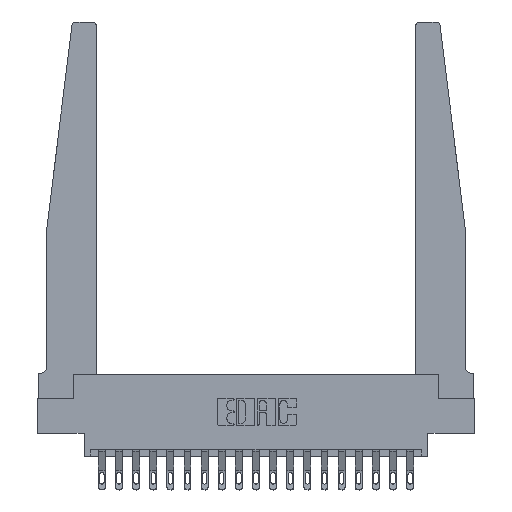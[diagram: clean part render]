
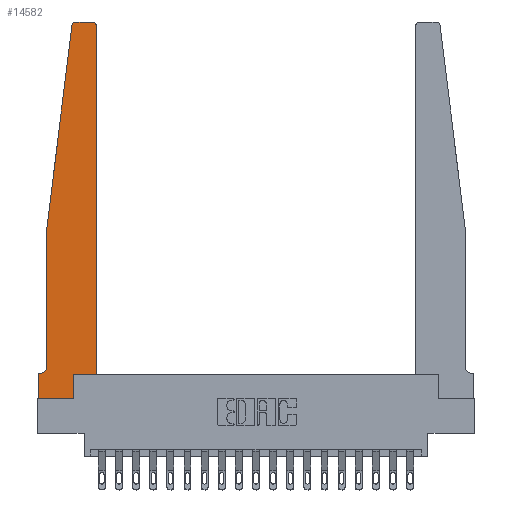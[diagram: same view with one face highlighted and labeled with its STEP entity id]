
A CAD part, top view. The second image highlights one B-rep face of the part: STEP entity #14582.
In plain terms, the highlighted planar face has unit normal (0, 0, 1).
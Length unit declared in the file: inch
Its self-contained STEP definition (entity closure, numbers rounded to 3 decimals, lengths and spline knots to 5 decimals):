
#494 = CARTESIAN_POINT ( 'NONE',  ( 0.425, 0.18, 0.37 ) ) ;
#512 = CARTESIAN_POINT ( 'NONE',  ( 0., 0., 0.37 ) ) ;
#1252 = CARTESIAN_POINT ( 'NONE',  ( 0.425, 0.18, 0.37 ) ) ;
#1759 = DIRECTION ( 'NONE',  ( 0., 1., 0. ) ) ;
#1803 = DIRECTION ( 'NONE',  ( 1., 0., 0. ) ) ;
#1852 = CARTESIAN_POINT ( 'NONE',  ( 0.2605, 0.18, 0.37 ) ) ;
#1976 = VERTEX_POINT ( 'NONE', #13450 ) ;
#2086 = DIRECTION ( 'NONE',  ( 0., 0., 1. ) ) ;
#2356 = VECTOR ( 'NONE', #1803, 39.37008 ) ;
#2367 = VECTOR ( 'NONE', #16394, 39.37008 ) ;
#2510 = DIRECTION ( 'NONE',  ( -1., 0., 0. ) ) ;
#2608 = CARTESIAN_POINT ( 'NONE',  ( 0.015, 0.2375, 0.37 ) ) ;
#2613 = VERTEX_POINT ( 'NONE', #1852 ) ;
#2911 = VERTEX_POINT ( 'NONE', #11051 ) ;
#3124 = ORIENTED_EDGE ( 'NONE', *, *, #18008, .T. ) ;
#3172 = CIRCLE ( 'NONE', #20982, 0.03 ) ;
#3353 = CARTESIAN_POINT ( 'NONE',  ( 0.065, 0.1875, 0.37 ) ) ;
#3414 = VERTEX_POINT ( 'NONE', #3780 ) ;
#3439 = ORIENTED_EDGE ( 'NONE', *, *, #6816, .T. ) ;
#3484 = EDGE_CURVE ( 'NONE', #9078, #5888, #3172, .T. ) ;
#3780 = CARTESIAN_POINT ( 'NONE',  ( 0.425, 0.18, 0.37 ) ) ;
#3910 = AXIS2_PLACEMENT_3D ( 'NONE', #19140, #8036, #21086 ) ;
#3924 = VECTOR ( 'NONE', #4923, 39.37008 ) ;
#3942 = CIRCLE ( 'NONE', #11148, 0.05 ) ;
#4830 = FACE_OUTER_BOUND ( 'NONE', #9101, .T. ) ;
#4867 = LINE ( 'NONE', #3353, #16237 ) ;
#4923 = DIRECTION ( 'NONE',  ( 0., -1., 0. ) ) ;
#5519 = VECTOR ( 'NONE', #19209, 39.37008 ) ;
#5888 = VERTEX_POINT ( 'NONE', #18949 ) ;
#6439 = ORIENTED_EDGE ( 'NONE', *, *, #17632, .T. ) ;
#6446 = PLANE ( 'NONE',  #6995 ) ;
#6758 = LINE ( 'NONE', #8273, #3924 ) ;
#6816 = EDGE_CURVE ( 'NONE', #17831, #2911, #14531, .T. ) ;
#6824 = VECTOR ( 'NONE', #8120, 39.37008 ) ;
#6889 = EDGE_CURVE ( 'NONE', #13131, #13969, #13159, .T. ) ;
#6995 = AXIS2_PLACEMENT_3D ( 'NONE', #12984, #9667, #11596 ) ;
#7030 = ORIENTED_EDGE ( 'NONE', *, *, #18365, .T. ) ;
#7770 = LINE ( 'NONE', #14387, #5519 ) ;
#7805 = DIRECTION ( 'NONE',  ( 0., 1., 0. ) ) ;
#8036 = DIRECTION ( 'NONE',  ( 0., 0., 1. ) ) ;
#8120 = DIRECTION ( 'NONE',  ( 0., -1., 0. ) ) ;
#8273 = CARTESIAN_POINT ( 'NONE',  ( 0.065, 1.25, 0.37 ) ) ;
#8353 = EDGE_CURVE ( 'NONE', #17542, #13131, #9708, .T. ) ;
#9044 = CARTESIAN_POINT ( 'NONE',  ( 0.425, 2.72, 0.37 ) ) ;
#9078 = VERTEX_POINT ( 'NONE', #9044 ) ;
#9101 = EDGE_LOOP ( 'NONE', ( #16746, #3439, #15639, #6439, #3124, #14637, #19939, #14296, #7030, #11857, #20374, #21070 ) ) ;
#9299 = EDGE_CURVE ( 'NONE', #2911, #1976, #10105, .T. ) ;
#9595 = DIRECTION ( 'NONE',  ( -1., 0., 0. ) ) ;
#9667 = DIRECTION ( 'NONE',  ( 0., 0., 1. ) ) ;
#9708 = LINE ( 'NONE', #17937, #6824 ) ;
#10077 = VERTEX_POINT ( 'NONE', #16934 ) ;
#10105 = LINE ( 'NONE', #12977, #2367 ) ;
#10882 = CARTESIAN_POINT ( 'NONE',  ( 0.2605, 0., 0.37 ) ) ;
#10960 = EDGE_CURVE ( 'NONE', #5888, #17831, #7770, .T. ) ;
#11051 = CARTESIAN_POINT ( 'NONE',  ( 0.24675, 2.72367, 0.37 ) ) ;
#11148 = AXIS2_PLACEMENT_3D ( 'NONE', #2608, #20522, #2510 ) ;
#11596 = DIRECTION ( 'NONE',  ( 1., 0., 0. ) ) ;
#11753 = CARTESIAN_POINT ( 'NONE',  ( 0.395, 2.72, 0.37 ) ) ;
#11759 = EDGE_CURVE ( 'NONE', #2613, #3414, #19674, .T. ) ;
#11763 = DIRECTION ( 'NONE',  ( 1., 0., 0. ) ) ;
#11855 = DIRECTION ( 'NONE',  ( 1., 0., 0. ) ) ;
#11857 = ORIENTED_EDGE ( 'NONE', *, *, #11759, .T. ) ;
#12224 = VECTOR ( 'NONE', #7805, 39.37008 ) ;
#12438 = CARTESIAN_POINT ( 'NONE',  ( 0.27653, 2.75, 0.37 ) ) ;
#12977 = CARTESIAN_POINT ( 'NONE',  ( 0.065, 1.25, 0.37 ) ) ;
#12984 = CARTESIAN_POINT ( 'NONE',  ( 0., 0.1875, 0.37 ) ) ;
#13131 = VERTEX_POINT ( 'NONE', #16788 ) ;
#13159 = LINE ( 'NONE', #512, #2356 ) ;
#13450 = CARTESIAN_POINT ( 'NONE',  ( 0.065, 1.25, 0.37 ) ) ;
#13969 = VERTEX_POINT ( 'NONE', #10882 ) ;
#14296 = ORIENTED_EDGE ( 'NONE', *, *, #6889, .T. ) ;
#14387 = CARTESIAN_POINT ( 'NONE',  ( 0.25, 2.75, 0.37 ) ) ;
#14531 = CIRCLE ( 'NONE', #3910, 0.03 ) ;
#14582 = ADVANCED_FACE ( 'NONE', ( #4830 ), #6446, .T. ) ;
#14637 = ORIENTED_EDGE ( 'NONE', *, *, #17065, .T. ) ;
#15042 = LINE ( 'NONE', #18255, #17616 ) ;
#15639 = ORIENTED_EDGE ( 'NONE', *, *, #9299, .T. ) ;
#15937 = LINE ( 'NONE', #1252, #12224 ) ;
#16237 = VECTOR ( 'NONE', #9595, 39.37008 ) ;
#16394 = DIRECTION ( 'NONE',  ( -0.122, -0.992, 0. ) ) ;
#16433 = CARTESIAN_POINT ( 'NONE',  ( 0.015, 0.1875, 0.37 ) ) ;
#16746 = ORIENTED_EDGE ( 'NONE', *, *, #10960, .T. ) ;
#16788 = CARTESIAN_POINT ( 'NONE',  ( 0., 0., 0.37 ) ) ;
#16934 = CARTESIAN_POINT ( 'NONE',  ( 0.065, 0.2375, 0.37 ) ) ;
#17065 = EDGE_CURVE ( 'NONE', #20777, #17542, #4867, .T. ) ;
#17542 = VERTEX_POINT ( 'NONE', #19815 ) ;
#17616 = VECTOR ( 'NONE', #1759, 39.37008 ) ;
#17632 = EDGE_CURVE ( 'NONE', #1976, #10077, #6758, .T. ) ;
#17831 = VERTEX_POINT ( 'NONE', #12438 ) ;
#17937 = CARTESIAN_POINT ( 'NONE',  ( 0., 0., 0.37 ) ) ;
#18008 = EDGE_CURVE ( 'NONE', #10077, #20777, #3942, .T. ) ;
#18193 = VECTOR ( 'NONE', #11763, 39.37008 ) ;
#18255 = CARTESIAN_POINT ( 'NONE',  ( 0.2605, 0.18, 0.37 ) ) ;
#18365 = EDGE_CURVE ( 'NONE', #13969, #2613, #15042, .T. ) ;
#18949 = CARTESIAN_POINT ( 'NONE',  ( 0.395, 2.75, 0.37 ) ) ;
#19115 = EDGE_CURVE ( 'NONE', #3414, #9078, #15937, .T. ) ;
#19140 = CARTESIAN_POINT ( 'NONE',  ( 0.27653, 2.72, 0.37 ) ) ;
#19209 = DIRECTION ( 'NONE',  ( -1., 0., 0. ) ) ;
#19674 = LINE ( 'NONE', #494, #18193 ) ;
#19815 = CARTESIAN_POINT ( 'NONE',  ( 0., 0.1875, 0.37 ) ) ;
#19939 = ORIENTED_EDGE ( 'NONE', *, *, #8353, .T. ) ;
#20374 = ORIENTED_EDGE ( 'NONE', *, *, #19115, .T. ) ;
#20522 = DIRECTION ( 'NONE',  ( 0., 0., -1. ) ) ;
#20777 = VERTEX_POINT ( 'NONE', #16433 ) ;
#20982 = AXIS2_PLACEMENT_3D ( 'NONE', #11753, #2086, #11855 ) ;
#21070 = ORIENTED_EDGE ( 'NONE', *, *, #3484, .T. ) ;
#21086 = DIRECTION ( 'NONE',  ( 1., 0., 0. ) ) ;
